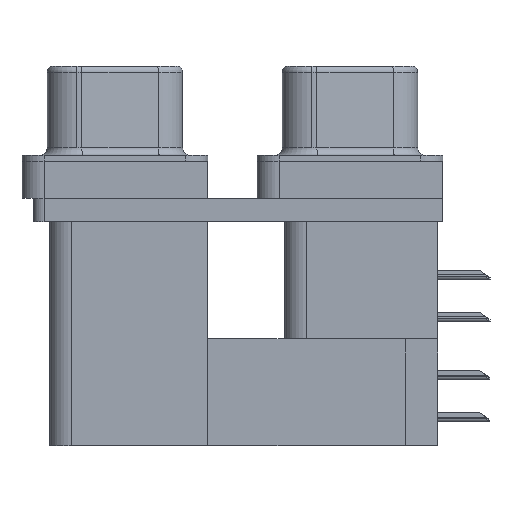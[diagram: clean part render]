
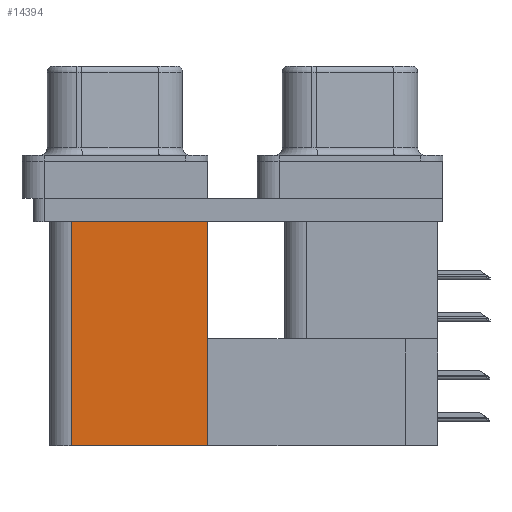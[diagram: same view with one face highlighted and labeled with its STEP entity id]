
A CAD part, left-side view. The second image highlights one B-rep face of the part: STEP entity #14394.
In plain terms, the highlighted planar face has unit normal (-1, 0, 0).
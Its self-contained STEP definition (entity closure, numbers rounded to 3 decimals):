
#31 = DIRECTION ( 'NONE',  ( 0., 0., 1. ) ) ;
#1378 = DIRECTION ( 'NONE',  ( 0., 1., 0. ) ) ;
#2536 = DIRECTION ( 'NONE',  ( 1., 0., 0. ) ) ;
#4384 = LINE ( 'NONE', #16714, #27876 ) ;
#4657 = VERTEX_POINT ( 'NONE', #21690 ) ;
#4748 = VERTEX_POINT ( 'NONE', #22882 ) ;
#9508 = VERTEX_POINT ( 'NONE', #11604 ) ;
#9793 = EDGE_CURVE ( 'NONE', #4657, #31502, #19093, .T. ) ;
#10863 = CARTESIAN_POINT ( 'NONE',  ( 3.7, 9.6, -2.5 ) ) ;
#10978 = ORIENTED_EDGE ( 'NONE', *, *, #14334, .T. ) ;
#11604 = CARTESIAN_POINT ( 'NONE',  ( 3.7, 9.6, -2.5 ) ) ;
#13507 = LINE ( 'NONE', #10863, #18802 ) ;
#13518 = ORIENTED_EDGE ( 'NONE', *, *, #20192, .T. ) ;
#13799 = CARTESIAN_POINT ( 'NONE',  ( 3.7, 18.8, -19.2 ) ) ;
#14334 = EDGE_CURVE ( 'NONE', #4657, #9508, #4384, .T. ) ;
#14394 = ADVANCED_FACE ( 'NONE', ( #14676 ), #32878, .F. ) ;
#14676 = FACE_OUTER_BOUND ( 'NONE', #21081, .T. ) ;
#15410 = LINE ( 'NONE', #34631, #28573 ) ;
#15866 = DIRECTION ( 'NONE',  ( 0., 1., 0. ) ) ;
#16714 = CARTESIAN_POINT ( 'NONE',  ( 3.7, 9.6, -19.2 ) ) ;
#18802 = VECTOR ( 'NONE', #1378, 1000. ) ;
#19093 = LINE ( 'NONE', #20223, #29000 ) ;
#20192 = EDGE_CURVE ( 'NONE', #9508, #4748, #13507, .T. ) ;
#20223 = CARTESIAN_POINT ( 'NONE',  ( 3.7, 9.6, -19.2 ) ) ;
#21081 = EDGE_LOOP ( 'NONE', ( #13518, #39748, #36989, #10978 ) ) ;
#21428 = EDGE_CURVE ( 'NONE', #31502, #4748, #15410, .T. ) ;
#21690 = CARTESIAN_POINT ( 'NONE',  ( 3.7, 9.6, -19.2 ) ) ;
#22882 = CARTESIAN_POINT ( 'NONE',  ( 3.7, 18.8, -2.5 ) ) ;
#23001 = DIRECTION ( 'NONE',  ( 0., 0., 1. ) ) ;
#23595 = CARTESIAN_POINT ( 'NONE',  ( 3.7, 9.6, -19.2 ) ) ;
#27210 = DIRECTION ( 'NONE',  ( 0., 0., -1. ) ) ;
#27876 = VECTOR ( 'NONE', #23001, 1000. ) ;
#28573 = VECTOR ( 'NONE', #31, 1000. ) ;
#29000 = VECTOR ( 'NONE', #15866, 1000. ) ;
#31502 = VERTEX_POINT ( 'NONE', #13799 ) ;
#32878 = PLANE ( 'NONE',  #38843 ) ;
#34631 = CARTESIAN_POINT ( 'NONE',  ( 3.7, 18.8, -19.2 ) ) ;
#36989 = ORIENTED_EDGE ( 'NONE', *, *, #9793, .F. ) ;
#38843 = AXIS2_PLACEMENT_3D ( 'NONE', #23595, #2536, #27210 ) ;
#39748 = ORIENTED_EDGE ( 'NONE', *, *, #21428, .F. ) ;
